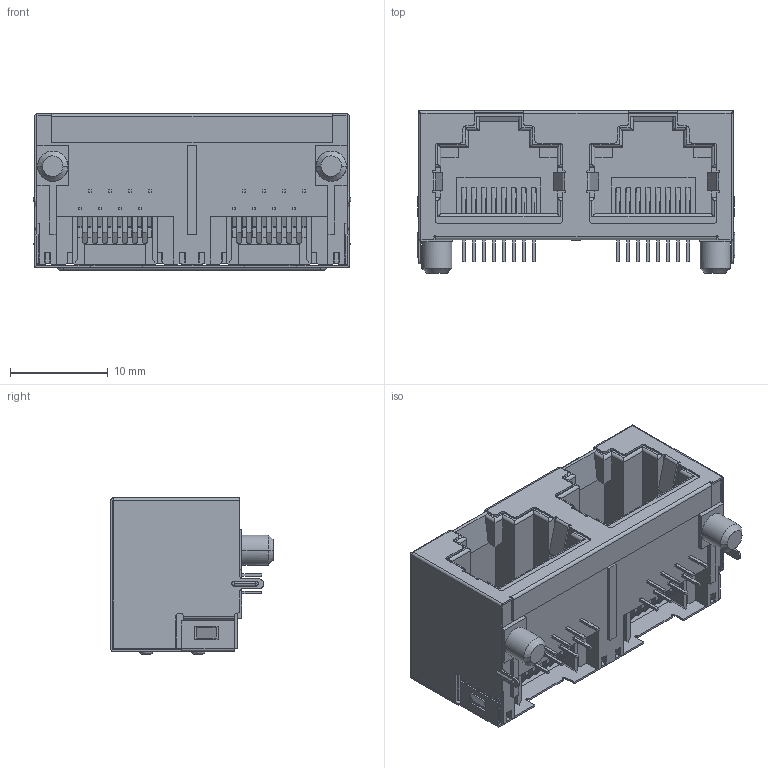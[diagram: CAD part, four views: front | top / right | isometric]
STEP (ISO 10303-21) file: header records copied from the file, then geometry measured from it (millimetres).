
FILE_DESCRIPTION (( 'STEP AP203' ), '1' );
FILE_NAME ('J6A028822N00112.STEP', '2020-03-17T18:08:06', ( '' ), ( '' ), 'SwSTEP 2.0', 'SolidWorks 2016', '' );
FILE_SCHEMA (( 'CONFIG_CONTROL_DESIGN' ));
Length unit declared in the file: millimetre
Products named in the file (4): J6A028822N00112; 6A Insulator; 6A Contacts; 6A Shield
Assembly tree (4 placements, depth 2):
  J6A028822N00112
    6A Insulator
    6A Contacts  x2
    6A Shield
Bounding box: 32.47 x 16.6 x 15.95 mm (x, y, z)
Volume: 2964.5 mm3; surface area: 8171.9 mm2
Topology: 18 solids, 18 shells, 1823 faces, 5021 edges, 3239 vertices
Faces by surface type: plane 1380, cylinder 415, bspline 23, cone 4, torus 1
Entity records: 52715 total; most frequent: CARTESIAN_POINT 12562, ORIENTED_EDGE 8778, DIRECTION 7477, EDGE_CURVE 4389, VECTOR 3319, LINE 3319, VERTEX_POINT 2831, AXIS2_PLACEMENT_3D 2079
